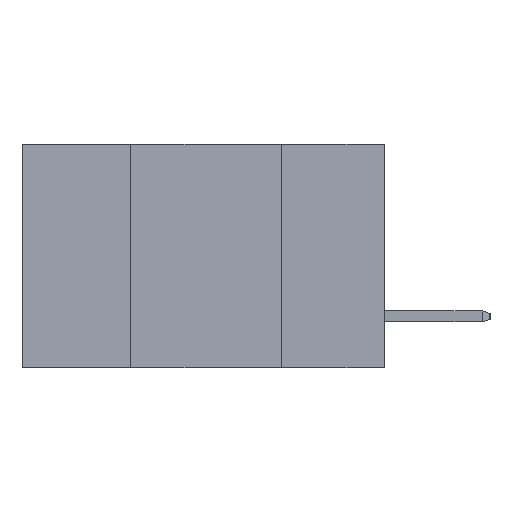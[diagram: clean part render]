
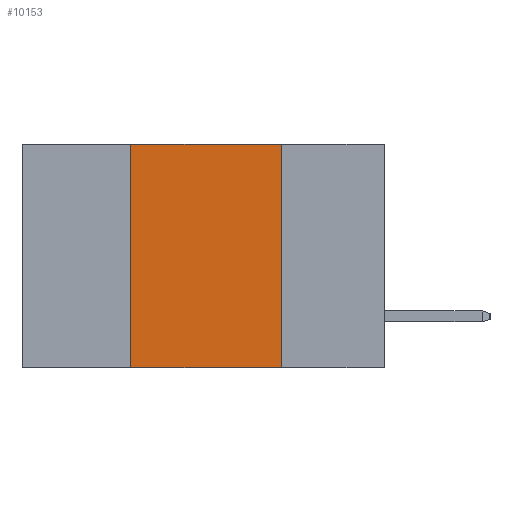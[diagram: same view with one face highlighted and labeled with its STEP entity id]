
A CAD part, left-side view. The second image highlights one B-rep face of the part: STEP entity #10153.
In plain terms, the highlighted planar face has unit normal (-1, 0, 0).
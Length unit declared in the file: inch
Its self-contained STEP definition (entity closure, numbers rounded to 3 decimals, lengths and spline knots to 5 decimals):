
#798 = CARTESIAN_POINT ( 'NONE',  ( 0., 0.6, -0.37 ) ) ;
#858 = CARTESIAN_POINT ( 'NONE',  ( 0., 0.42, 0. ) ) ;
#947 = VERTEX_POINT ( 'NONE', #8216 ) ;
#1886 = ORIENTED_EDGE ( 'NONE', *, *, #12758, .T. ) ;
#2033 = DIRECTION ( 'NONE',  ( 0., -1., 0. ) ) ;
#2095 = CARTESIAN_POINT ( 'NONE',  ( 0., 0.6, 0. ) ) ;
#2097 = LINE ( 'NONE', #798, #12919 ) ;
#2694 = DIRECTION ( 'NONE',  ( 1., 0., 0. ) ) ;
#2704 = VERTEX_POINT ( 'NONE', #7136 ) ;
#3249 = ORIENTED_EDGE ( 'NONE', *, *, #9920, .F. ) ;
#4932 = CARTESIAN_POINT ( 'NONE',  ( 0., 0.17, -0.37 ) ) ;
#6157 = CARTESIAN_POINT ( 'NONE',  ( 0., 0.42, -0.37 ) ) ;
#6507 = ORIENTED_EDGE ( 'NONE', *, *, #11812, .F. ) ;
#6940 = LINE ( 'NONE', #6157, #7389 ) ;
#7136 = CARTESIAN_POINT ( 'NONE',  ( 0., 0.17, 0. ) ) ;
#7389 = VECTOR ( 'NONE', #13299, 39.37008 ) ;
#8216 = CARTESIAN_POINT ( 'NONE',  ( 0., 0.42, -0.37 ) ) ;
#9920 = EDGE_CURVE ( 'NONE', #2704, #16534, #18109, .T. ) ;
#10153 = ADVANCED_FACE ( 'NONE', ( #17450 ), #15390, .F. ) ;
#10498 = EDGE_CURVE ( 'NONE', #14751, #2704, #11660, .T. ) ;
#11185 = CARTESIAN_POINT ( 'NONE',  ( 0., 0.6, 0. ) ) ;
#11252 = CARTESIAN_POINT ( 'NONE',  ( 0., 0.17, -0.37 ) ) ;
#11645 = ORIENTED_EDGE ( 'NONE', *, *, #10498, .F. ) ;
#11660 = LINE ( 'NONE', #2095, #12092 ) ;
#11812 = EDGE_CURVE ( 'NONE', #947, #14751, #6940, .T. ) ;
#11985 = DIRECTION ( 'NONE',  ( 0., 0., -1. ) ) ;
#12092 = VECTOR ( 'NONE', #2033, 39.37008 ) ;
#12131 = DIRECTION ( 'NONE',  ( 0., -1., 0. ) ) ;
#12592 = DIRECTION ( 'NONE',  ( 0., 0., -1. ) ) ;
#12758 = EDGE_CURVE ( 'NONE', #947, #16534, #2097, .T. ) ;
#12919 = VECTOR ( 'NONE', #12131, 39.37008 ) ;
#13299 = DIRECTION ( 'NONE',  ( 0., 0., 1. ) ) ;
#14478 = AXIS2_PLACEMENT_3D ( 'NONE', #11185, #2694, #12592 ) ;
#14751 = VERTEX_POINT ( 'NONE', #858 ) ;
#15390 = PLANE ( 'NONE',  #14478 ) ;
#16534 = VERTEX_POINT ( 'NONE', #11252 ) ;
#17011 = EDGE_LOOP ( 'NONE', ( #3249, #11645, #6507, #1886 ) ) ;
#17450 = FACE_OUTER_BOUND ( 'NONE', #17011, .T. ) ;
#17678 = VECTOR ( 'NONE', #11985, 39.37008 ) ;
#18109 = LINE ( 'NONE', #4932, #17678 ) ;
